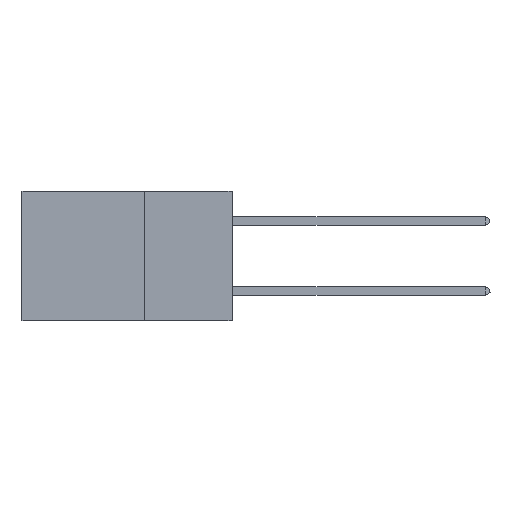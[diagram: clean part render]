
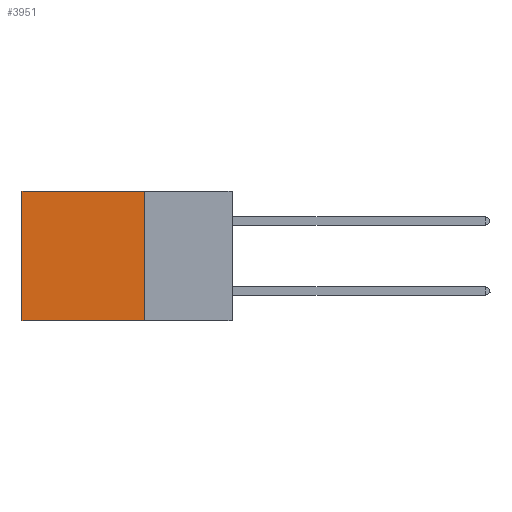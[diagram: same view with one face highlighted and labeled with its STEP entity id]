
A CAD part, left-side view. The second image highlights one B-rep face of the part: STEP entity #3951.
In plain terms, the highlighted planar face has unit normal (-1, 0, 0).
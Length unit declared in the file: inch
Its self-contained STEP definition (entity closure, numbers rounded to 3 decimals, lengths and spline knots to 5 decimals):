
#2388 = ORIENTED_EDGE ( 'NONE', *, *, #7579, .T. ) ;
#2462 = CARTESIAN_POINT ( 'NONE',  ( 0.2875, 0.6, -0.37 ) ) ;
#3543 = VERTEX_POINT ( 'NONE', #12140 ) ;
#3951 = ADVANCED_FACE ( 'NONE', ( #22140 ), #14230, .F. ) ;
#5252 = AXIS2_PLACEMENT_3D ( 'NONE', #6172, #24134, #10082 ) ;
#6172 = CARTESIAN_POINT ( 'NONE',  ( 0.2875, 0.25, 0. ) ) ;
#6486 = VECTOR ( 'NONE', #8882, 39.37008 ) ;
#6900 = CARTESIAN_POINT ( 'NONE',  ( 0.2875, 0.25, 0. ) ) ;
#7579 = EDGE_CURVE ( 'NONE', #8753, #16610, #24546, .T. ) ;
#8510 = EDGE_CURVE ( 'NONE', #3543, #16610, #8859, .T. ) ;
#8746 = DIRECTION ( 'NONE',  ( 0., 0., -1. ) ) ;
#8753 = VERTEX_POINT ( 'NONE', #21477 ) ;
#8859 = LINE ( 'NONE', #11206, #13589 ) ;
#8882 = DIRECTION ( 'NONE',  ( 0., 0., -1. ) ) ;
#10082 = DIRECTION ( 'NONE',  ( 0., 0., -1. ) ) ;
#11029 = CARTESIAN_POINT ( 'NONE',  ( 0.2875, 0.6, 0. ) ) ;
#11206 = CARTESIAN_POINT ( 'NONE',  ( 0.2875, 0.25, -0.37 ) ) ;
#11373 = ORIENTED_EDGE ( 'NONE', *, *, #13030, .F. ) ;
#11811 = DIRECTION ( 'NONE',  ( 0., 1., 0. ) ) ;
#12140 = CARTESIAN_POINT ( 'NONE',  ( 0.2875, 0.25, -0.37 ) ) ;
#12392 = VECTOR ( 'NONE', #11811, 39.37008 ) ;
#13030 = EDGE_CURVE ( 'NONE', #18129, #3543, #17045, .T. ) ;
#13589 = VECTOR ( 'NONE', #23345, 39.37008 ) ;
#14230 = PLANE ( 'NONE',  #5252 ) ;
#15021 = EDGE_LOOP ( 'NONE', ( #2388, #16206, #11373, #15905 ) ) ;
#15024 = CARTESIAN_POINT ( 'NONE',  ( 0.2875, 0.25, 0. ) ) ;
#15491 = LINE ( 'NONE', #21717, #12392 ) ;
#15905 = ORIENTED_EDGE ( 'NONE', *, *, #22882, .T. ) ;
#16206 = ORIENTED_EDGE ( 'NONE', *, *, #8510, .F. ) ;
#16610 = VERTEX_POINT ( 'NONE', #2462 ) ;
#17045 = LINE ( 'NONE', #6900, #6486 ) ;
#18129 = VERTEX_POINT ( 'NONE', #15024 ) ;
#19524 = VECTOR ( 'NONE', #8746, 39.37008 ) ;
#21477 = CARTESIAN_POINT ( 'NONE',  ( 0.2875, 0.6, 0. ) ) ;
#21717 = CARTESIAN_POINT ( 'NONE',  ( 0.2875, 0.25, 0. ) ) ;
#22140 = FACE_OUTER_BOUND ( 'NONE', #15021, .T. ) ;
#22882 = EDGE_CURVE ( 'NONE', #18129, #8753, #15491, .T. ) ;
#23345 = DIRECTION ( 'NONE',  ( 0., 1., 0. ) ) ;
#24134 = DIRECTION ( 'NONE',  ( 1., 0., 0. ) ) ;
#24546 = LINE ( 'NONE', #11029, #19524 ) ;
